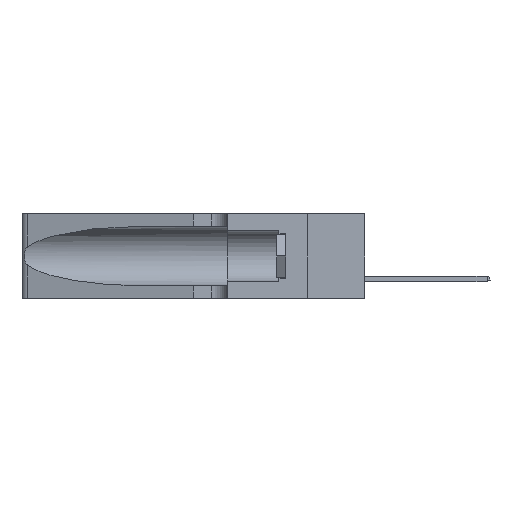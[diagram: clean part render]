
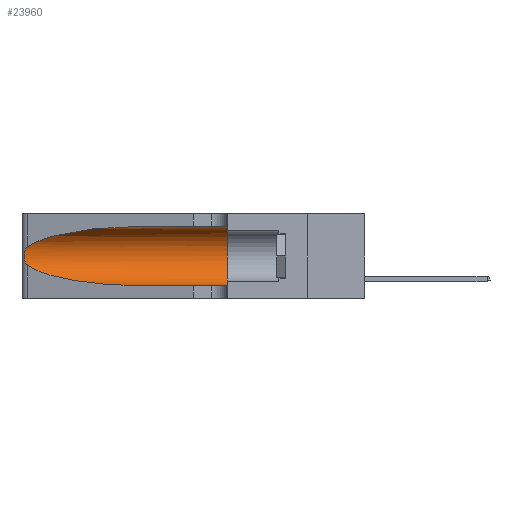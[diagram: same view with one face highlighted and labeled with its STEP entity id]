
A CAD part, left-side view. The second image highlights one B-rep face of the part: STEP entity #23960.
In plain terms, the highlighted cylindrical face has radius 3.308 mm (diameter 6.617 mm), a partial arc.
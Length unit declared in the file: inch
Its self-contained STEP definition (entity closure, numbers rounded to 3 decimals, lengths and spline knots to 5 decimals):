
#1004 = CARTESIAN_POINT ( 'NONE',  ( 0.26075, 1.23896, 0.178 ) ) ;
#1320 = CARTESIAN_POINT ( 'NONE',  ( 0.25555, 1.22994, 0.2215 ) ) ;
#1484 = CARTESIAN_POINT ( 'NONE',  ( 0.26018, 1.23835, 0.19895 ) ) ;
#2144 = CARTESIAN_POINT ( 'NONE',  ( 0.1305, 1.61858, 0.185 ) ) ;
#2819 = DIRECTION ( 'NONE',  ( 0., 0., -1. ) ) ;
#3070 = DIRECTION ( 'NONE',  ( 0., 1., 0. ) ) ;
#4809 = VECTOR ( 'NONE', #12664, 39.37008 ) ;
#5071 = CARTESIAN_POINT ( 'NONE',  ( 0.25789, 1.23486, 0.15765 ) ) ;
#5338 = CARTESIAN_POINT ( 'NONE',  ( 0.1305, 1.61858, 0.05475 ) ) ;
#5583 = CARTESIAN_POINT ( 'NONE',  ( 0.18966, 0.96281, 0.31525 ) ) ;
#6150 = ORIENTED_EDGE ( 'NONE', *, *, #29949, .F. ) ;
#6496 = EDGE_CURVE ( 'NONE', #46761, #34384, #16991, .T. ) ;
#6862 =( BOUNDED_CURVE ( )  B_SPLINE_CURVE ( 3, ( #46787, #13071, #16824, #24417 ),
 .UNSPECIFIED., .F., .T. ) 
 B_SPLINE_CURVE_WITH_KNOTS ( ( 4, 4 ),
 ( 3.44316, 4.71239 ),
 .UNSPECIFIED. ) 
 CURVE ( )  GEOMETRIC_REPRESENTATION_ITEM ( )  RATIONAL_B_SPLINE_CURVE ( ( 1., 0.87, 0.87, 1. ) ) 
 REPRESENTATION_ITEM ( '' )  );
#8981 = CARTESIAN_POINT ( 'NONE',  ( 0.26075, 1.23896, 0.19203 ) ) ;
#9129 = VECTOR ( 'NONE', #32927, 39.37008 ) ;
#9479 = DIRECTION ( 'NONE',  ( 0., -1., 0. ) ) ;
#10121 = ORIENTED_EDGE ( 'NONE', *, *, #36892, .T. ) ;
#12664 = DIRECTION ( 'NONE',  ( 0., -1., 0. ) ) ;
#12740 = CARTESIAN_POINT ( 'NONE',  ( 0.25856, 1.23593, 0.16098 ) ) ;
#12904 = EDGE_CURVE ( 'NONE', #15862, #42921, #30017, .T. ) ;
#13071 = CARTESIAN_POINT ( 'NONE',  ( 0.2373, 1.15595, 0.08982 ) ) ;
#14134 = CARTESIAN_POINT ( 'NONE',  ( 0.1305, 0.72297, 0.05475 ) ) ;
#14307 = CARTESIAN_POINT ( 'NONE',  ( 0.1305, 0.35, 0.185 ) ) ;
#15477 =( BOUNDED_CURVE ( )  B_SPLINE_CURVE ( 3, ( #39218, #5583, #34961, #31803 ),
 .UNSPECIFIED., .F., .T. ) 
 B_SPLINE_CURVE_WITH_KNOTS ( ( 4, 4 ),
 ( 1.5708, 2.84003 ),
 .UNSPECIFIED. ) 
 CURVE ( )  GEOMETRIC_REPRESENTATION_ITEM ( )  RATIONAL_B_SPLINE_CURVE ( ( 1., 0.87, 0.87, 1. ) ) 
 REPRESENTATION_ITEM ( '' )  );
#15862 = VERTEX_POINT ( 'NONE', #14134 ) ;
#15991 = CARTESIAN_POINT ( 'NONE',  ( 0.26017, 1.23833, 0.17102 ) ) ;
#16501 = EDGE_CURVE ( 'NONE', #34384, #15862, #6862, .T. ) ;
#16737 = EDGE_CURVE ( 'NONE', #46067, #42921, #33183, .T. ) ;
#16824 = CARTESIAN_POINT ( 'NONE',  ( 0.18966, 0.96281, 0.05475 ) ) ;
#16991 = B_SPLINE_CURVE_WITH_KNOTS ( 'NONE', 3,
 ( #18813, #1320, #23245, #31284, #46117, #1484, #8981, #1004, #15991, #12740, #5071, #23912, #27363, #35239 ),
 .UNSPECIFIED., .F., .F.,
 ( 4, 2, 2, 2, 2, 2, 4 ),
 ( 0., 0.00027, 0.00053, 0.00107, 0.0016, 0.00187, 0.00214 ),
 .UNSPECIFIED. ) ;
#18809 = CARTESIAN_POINT ( 'NONE',  ( 0.1305, 0.72297, 0.31525 ) ) ;
#18813 = CARTESIAN_POINT ( 'NONE',  ( 0.25487, 1.22718, 0.22369 ) ) ;
#18999 = AXIS2_PLACEMENT_3D ( 'NONE', #2144, #9479, #2819 ) ;
#21894 = ORIENTED_EDGE ( 'NONE', *, *, #16737, .F. ) ;
#22250 = AXIS2_PLACEMENT_3D ( 'NONE', #14307, #3070, #29592 ) ;
#22476 = CARTESIAN_POINT ( 'NONE',  ( 0.1305, 0.35, 0.05475 ) ) ;
#23245 = CARTESIAN_POINT ( 'NONE',  ( 0.25639, 1.23184, 0.21858 ) ) ;
#23801 = CARTESIAN_POINT ( 'NONE',  ( 0.25487, 1.22718, 0.14631 ) ) ;
#23912 = CARTESIAN_POINT ( 'NONE',  ( 0.25639, 1.23186, 0.15144 ) ) ;
#23960 = ADVANCED_FACE ( 'NONE', ( #40196 ), #34249, .F. ) ;
#24417 = CARTESIAN_POINT ( 'NONE',  ( 0.1305, 0.72297, 0.05475 ) ) ;
#27363 = CARTESIAN_POINT ( 'NONE',  ( 0.25555, 1.22993, 0.14849 ) ) ;
#29592 = DIRECTION ( 'NONE',  ( 0., 0., 1. ) ) ;
#29949 = EDGE_CURVE ( 'NONE', #42073, #46067, #39099, .T. ) ;
#30017 = LINE ( 'NONE', #5338, #4809 ) ;
#31284 = CARTESIAN_POINT ( 'NONE',  ( 0.25787, 1.23484, 0.2124 ) ) ;
#31803 = CARTESIAN_POINT ( 'NONE',  ( 0.25487, 1.22718, 0.22369 ) ) ;
#31932 = EDGE_LOOP ( 'NONE', ( #10121, #39572, #38684, #47710, #21894, #6150 ) ) ;
#32927 = DIRECTION ( 'NONE',  ( 0., -1., 0. ) ) ;
#33183 = CIRCLE ( 'NONE', #22250, 0.13025 ) ;
#34249 = CYLINDRICAL_SURFACE ( 'NONE', #18999, 0.13025 ) ;
#34384 = VERTEX_POINT ( 'NONE', #23801 ) ;
#34961 = CARTESIAN_POINT ( 'NONE',  ( 0.2373, 1.15595, 0.28018 ) ) ;
#35239 = CARTESIAN_POINT ( 'NONE',  ( 0.25487, 1.22718, 0.14631 ) ) ;
#36892 = EDGE_CURVE ( 'NONE', #42073, #46761, #15477, .T. ) ;
#37351 = CARTESIAN_POINT ( 'NONE',  ( 0.1305, 1.61858, 0.31525 ) ) ;
#38684 = ORIENTED_EDGE ( 'NONE', *, *, #16501, .T. ) ;
#39024 = CARTESIAN_POINT ( 'NONE',  ( 0.1305, 0.35, 0.31525 ) ) ;
#39099 = LINE ( 'NONE', #37351, #9129 ) ;
#39218 = CARTESIAN_POINT ( 'NONE',  ( 0.1305, 0.72297, 0.31525 ) ) ;
#39572 = ORIENTED_EDGE ( 'NONE', *, *, #6496, .T. ) ;
#39982 = CARTESIAN_POINT ( 'NONE',  ( 0.25487, 1.22718, 0.22369 ) ) ;
#40196 = FACE_OUTER_BOUND ( 'NONE', #31932, .T. ) ;
#42073 = VERTEX_POINT ( 'NONE', #18809 ) ;
#42921 = VERTEX_POINT ( 'NONE', #22476 ) ;
#46067 = VERTEX_POINT ( 'NONE', #39024 ) ;
#46117 = CARTESIAN_POINT ( 'NONE',  ( 0.25854, 1.2359, 0.20912 ) ) ;
#46761 = VERTEX_POINT ( 'NONE', #39982 ) ;
#46787 = CARTESIAN_POINT ( 'NONE',  ( 0.25487, 1.22718, 0.14631 ) ) ;
#47710 = ORIENTED_EDGE ( 'NONE', *, *, #12904, .T. ) ;
